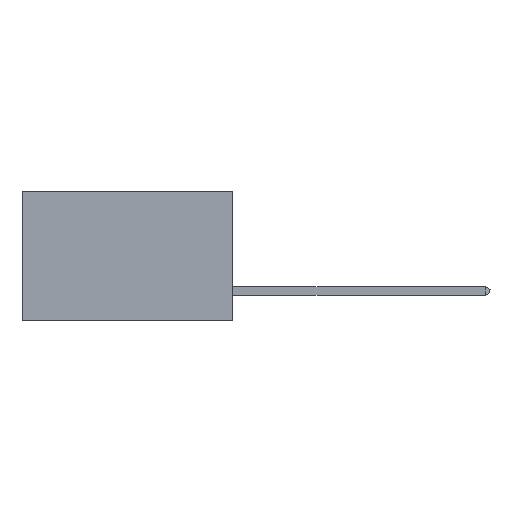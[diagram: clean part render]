
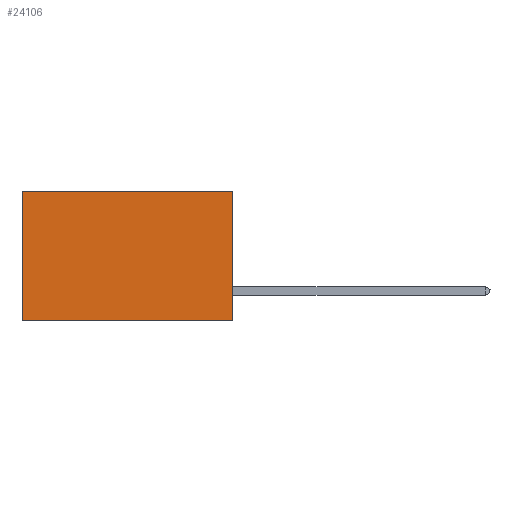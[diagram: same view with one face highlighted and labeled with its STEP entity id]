
A CAD part, left-side view. The second image highlights one B-rep face of the part: STEP entity #24106.
In plain terms, the highlighted planar face has unit normal (-1, 0, 0).
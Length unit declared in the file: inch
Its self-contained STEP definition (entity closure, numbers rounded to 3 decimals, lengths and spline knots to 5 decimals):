
#472 = LINE ( 'NONE', #21738, #38832 ) ;
#1393 = VERTEX_POINT ( 'NONE', #1773 ) ;
#1773 = CARTESIAN_POINT ( 'NONE',  ( 0.2875, 0.6, -0.37 ) ) ;
#1866 = ORIENTED_EDGE ( 'NONE', *, *, #8671, .T. ) ;
#2394 = CARTESIAN_POINT ( 'NONE',  ( 0.2875, 0., 0. ) ) ;
#2822 = DIRECTION ( 'NONE',  ( 0., 0., -1. ) ) ;
#3274 = VECTOR ( 'NONE', #35466, 39.37008 ) ;
#8182 = ORIENTED_EDGE ( 'NONE', *, *, #31891, .F. ) ;
#8451 = CARTESIAN_POINT ( 'NONE',  ( 0.2875, 0.6, 0. ) ) ;
#8671 = EDGE_CURVE ( 'NONE', #36402, #1393, #11311, .T. ) ;
#9479 = VERTEX_POINT ( 'NONE', #20960 ) ;
#10713 = VERTEX_POINT ( 'NONE', #15408 ) ;
#11311 = LINE ( 'NONE', #8451, #22214 ) ;
#12773 = CARTESIAN_POINT ( 'NONE',  ( 0.2875, 0.6, 0. ) ) ;
#14463 = DIRECTION ( 'NONE',  ( 1., 0., 0. ) ) ;
#15408 = CARTESIAN_POINT ( 'NONE',  ( 0.2875, 0., 0. ) ) ;
#16074 = LINE ( 'NONE', #20872, #27112 ) ;
#17817 = EDGE_CURVE ( 'NONE', #9479, #1393, #25658, .T. ) ;
#18825 = EDGE_CURVE ( 'NONE', #10713, #36402, #16074, .T. ) ;
#19281 = FACE_OUTER_BOUND ( 'NONE', #20733, .T. ) ;
#20733 = EDGE_LOOP ( 'NONE', ( #1866, #25231, #8182, #28974 ) ) ;
#20872 = CARTESIAN_POINT ( 'NONE',  ( 0.2875, 0., 0. ) ) ;
#20960 = CARTESIAN_POINT ( 'NONE',  ( 0.2875, 0., -0.37 ) ) ;
#21738 = CARTESIAN_POINT ( 'NONE',  ( 0.2875, 0., 0. ) ) ;
#22214 = VECTOR ( 'NONE', #33334, 39.37008 ) ;
#22527 = CARTESIAN_POINT ( 'NONE',  ( 0.2875, 0., -0.37 ) ) ;
#24106 = ADVANCED_FACE ( 'NONE', ( #19281 ), #24110, .F. ) ;
#24110 = PLANE ( 'NONE',  #36059 ) ;
#25231 = ORIENTED_EDGE ( 'NONE', *, *, #17817, .F. ) ;
#25658 = LINE ( 'NONE', #22527, #3274 ) ;
#27112 = VECTOR ( 'NONE', #40062, 39.37008 ) ;
#28974 = ORIENTED_EDGE ( 'NONE', *, *, #18825, .T. ) ;
#30659 = DIRECTION ( 'NONE',  ( 0., 0., -1. ) ) ;
#31891 = EDGE_CURVE ( 'NONE', #10713, #9479, #472, .T. ) ;
#33334 = DIRECTION ( 'NONE',  ( 0., 0., -1. ) ) ;
#35466 = DIRECTION ( 'NONE',  ( 0., 1., 0. ) ) ;
#36059 = AXIS2_PLACEMENT_3D ( 'NONE', #2394, #14463, #30659 ) ;
#36402 = VERTEX_POINT ( 'NONE', #12773 ) ;
#38832 = VECTOR ( 'NONE', #2822, 39.37008 ) ;
#40062 = DIRECTION ( 'NONE',  ( 0., 1., 0. ) ) ;
